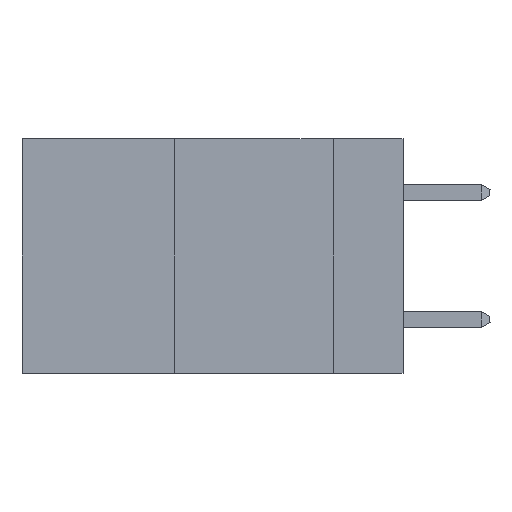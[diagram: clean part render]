
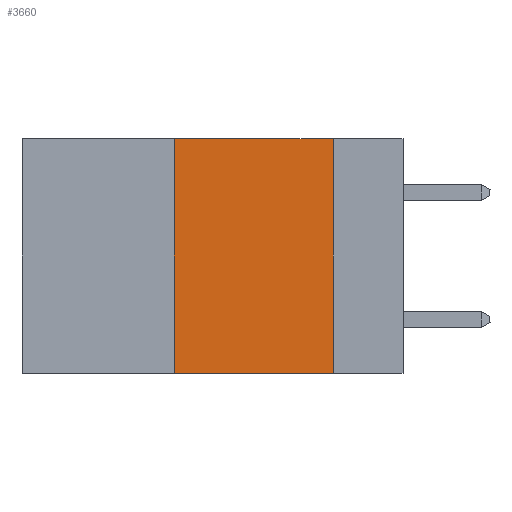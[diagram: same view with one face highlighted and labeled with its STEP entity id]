
A CAD part, left-side view. The second image highlights one B-rep face of the part: STEP entity #3660.
In plain terms, the highlighted planar face has unit normal (-1, 0, 0).
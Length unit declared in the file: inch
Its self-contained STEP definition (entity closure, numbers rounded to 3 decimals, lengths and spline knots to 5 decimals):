
#215 = ORIENTED_EDGE ( 'NONE', *, *, #560, .F. ) ;
#300 = EDGE_LOOP ( 'NONE', ( #6855, #5848, #215, #11940 ) ) ;
#560 = EDGE_CURVE ( 'NONE', #2472, #4553, #6931, .T. ) ;
#662 = VECTOR ( 'NONE', #10191, 39.37008 ) ;
#1079 = LINE ( 'NONE', #15320, #662 ) ;
#1582 = CARTESIAN_POINT ( 'NONE',  ( 0., 0.6, 0. ) ) ;
#2472 = VERTEX_POINT ( 'NONE', #5494 ) ;
#2848 = EDGE_CURVE ( 'NONE', #15687, #9041, #12775, .T. ) ;
#3660 = ADVANCED_FACE ( 'NONE', ( #13568 ), #14713, .F. ) ;
#3673 = CARTESIAN_POINT ( 'NONE',  ( 0., 0.11, 0. ) ) ;
#4553 = VERTEX_POINT ( 'NONE', #4975 ) ;
#4975 = CARTESIAN_POINT ( 'NONE',  ( 0., 0.36, 0. ) ) ;
#5494 = CARTESIAN_POINT ( 'NONE',  ( 0., 0.36, -0.37 ) ) ;
#5848 = ORIENTED_EDGE ( 'NONE', *, *, #14530, .F. ) ;
#6570 = VECTOR ( 'NONE', #8013, 39.37008 ) ;
#6855 = ORIENTED_EDGE ( 'NONE', *, *, #2848, .F. ) ;
#6926 = CARTESIAN_POINT ( 'NONE',  ( 0., 0.6, 0. ) ) ;
#6931 = LINE ( 'NONE', #8008, #13454 ) ;
#7965 = DIRECTION ( 'NONE',  ( 0., 0., 1. ) ) ;
#8008 = CARTESIAN_POINT ( 'NONE',  ( 0., 0.36, 0. ) ) ;
#8013 = DIRECTION ( 'NONE',  ( 0., -1., 0. ) ) ;
#8261 = DIRECTION ( 'NONE',  ( 0., 0., -1. ) ) ;
#8742 = EDGE_CURVE ( 'NONE', #2472, #9041, #1079, .T. ) ;
#9041 = VERTEX_POINT ( 'NONE', #15817 ) ;
#10051 = LINE ( 'NONE', #1582, #6570 ) ;
#10191 = DIRECTION ( 'NONE',  ( 0., -1., 0. ) ) ;
#11452 = DIRECTION ( 'NONE',  ( 0., 0., -1. ) ) ;
#11940 = ORIENTED_EDGE ( 'NONE', *, *, #8742, .T. ) ;
#12775 = LINE ( 'NONE', #3673, #16592 ) ;
#12902 = CARTESIAN_POINT ( 'NONE',  ( 0., 0.11, 0. ) ) ;
#13454 = VECTOR ( 'NONE', #7965, 39.37008 ) ;
#13568 = FACE_OUTER_BOUND ( 'NONE', #300, .T. ) ;
#14336 = AXIS2_PLACEMENT_3D ( 'NONE', #6926, #15981, #8261 ) ;
#14530 = EDGE_CURVE ( 'NONE', #4553, #15687, #10051, .T. ) ;
#14713 = PLANE ( 'NONE',  #14336 ) ;
#15320 = CARTESIAN_POINT ( 'NONE',  ( 0., 0.6, -0.37 ) ) ;
#15687 = VERTEX_POINT ( 'NONE', #12902 ) ;
#15817 = CARTESIAN_POINT ( 'NONE',  ( 0., 0.11, -0.37 ) ) ;
#15981 = DIRECTION ( 'NONE',  ( 1., 0., 0. ) ) ;
#16592 = VECTOR ( 'NONE', #11452, 39.37008 ) ;
